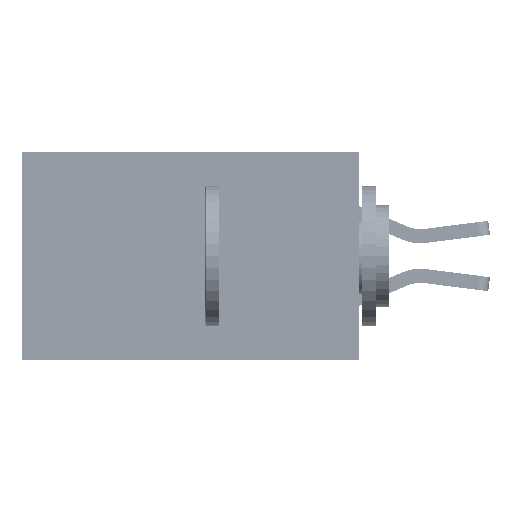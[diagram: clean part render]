
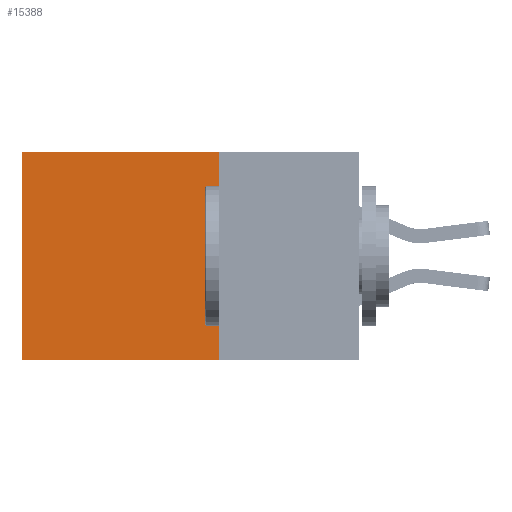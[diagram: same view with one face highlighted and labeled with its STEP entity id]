
A CAD part, left-side view. The second image highlights one B-rep face of the part: STEP entity #15388.
In plain terms, the highlighted planar face has unit normal (-1, 0, 0).
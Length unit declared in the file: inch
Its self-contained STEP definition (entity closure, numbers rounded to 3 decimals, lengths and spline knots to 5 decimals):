
#2555 = VECTOR ( 'NONE', #44380, 39.37008 ) ;
#2696 = DIRECTION ( 'NONE',  ( 0., 0., -1. ) ) ;
#3706 = CARTESIAN_POINT ( 'NONE',  ( 0.2875, 0.25, -0.37 ) ) ;
#4958 = ORIENTED_EDGE ( 'NONE', *, *, #18254, .T. ) ;
#5442 = LINE ( 'NONE', #25404, #36274 ) ;
#5520 = VECTOR ( 'NONE', #9793, 39.37008 ) ;
#5930 = DIRECTION ( 'NONE',  ( 0., 0., -1. ) ) ;
#6795 = LINE ( 'NONE', #29611, #5520 ) ;
#7772 = CARTESIAN_POINT ( 'NONE',  ( 0.2875, 0.25, 0. ) ) ;
#7810 = VECTOR ( 'NONE', #2696, 39.37008 ) ;
#8181 = LINE ( 'NONE', #40321, #2555 ) ;
#9793 = DIRECTION ( 'NONE',  ( 0., 1., 0. ) ) ;
#11412 = FACE_OUTER_BOUND ( 'NONE', #36737, .T. ) ;
#14807 = CARTESIAN_POINT ( 'NONE',  ( 0.2875, 0.6, -0.37 ) ) ;
#15388 = ADVANCED_FACE ( 'NONE', ( #11412 ), #47715, .F. ) ;
#18254 = EDGE_CURVE ( 'NONE', #35425, #21962, #35469, .T. ) ;
#20022 = CARTESIAN_POINT ( 'NONE',  ( 0.2875, 0.25, 0. ) ) ;
#21962 = VERTEX_POINT ( 'NONE', #14807 ) ;
#24380 = ORIENTED_EDGE ( 'NONE', *, *, #27874, .F. ) ;
#25404 = CARTESIAN_POINT ( 'NONE',  ( 0.2875, 0.25, 0. ) ) ;
#27874 = EDGE_CURVE ( 'NONE', #33998, #44097, #5442, .T. ) ;
#29066 = CARTESIAN_POINT ( 'NONE',  ( 0.2875, 0.6, 0. ) ) ;
#29611 = CARTESIAN_POINT ( 'NONE',  ( 0.2875, 0.25, 0. ) ) ;
#29709 = CARTESIAN_POINT ( 'NONE',  ( 0.2875, 0.6, 0. ) ) ;
#33998 = VERTEX_POINT ( 'NONE', #20022 ) ;
#35425 = VERTEX_POINT ( 'NONE', #29066 ) ;
#35469 = LINE ( 'NONE', #29709, #7810 ) ;
#36248 = DIRECTION ( 'NONE',  ( 1., 0., 0. ) ) ;
#36274 = VECTOR ( 'NONE', #5930, 39.37008 ) ;
#36737 = EDGE_LOOP ( 'NONE', ( #4958, #42398, #24380, #49275 ) ) ;
#40321 = CARTESIAN_POINT ( 'NONE',  ( 0.2875, 0.25, -0.37 ) ) ;
#41502 = EDGE_CURVE ( 'NONE', #44097, #21962, #8181, .T. ) ;
#41900 = AXIS2_PLACEMENT_3D ( 'NONE', #7772, #36248, #51814 ) ;
#42398 = ORIENTED_EDGE ( 'NONE', *, *, #41502, .F. ) ;
#44097 = VERTEX_POINT ( 'NONE', #3706 ) ;
#44380 = DIRECTION ( 'NONE',  ( 0., 1., 0. ) ) ;
#45663 = EDGE_CURVE ( 'NONE', #33998, #35425, #6795, .T. ) ;
#47715 = PLANE ( 'NONE',  #41900 ) ;
#49275 = ORIENTED_EDGE ( 'NONE', *, *, #45663, .T. ) ;
#51814 = DIRECTION ( 'NONE',  ( 0., 0., -1. ) ) ;
